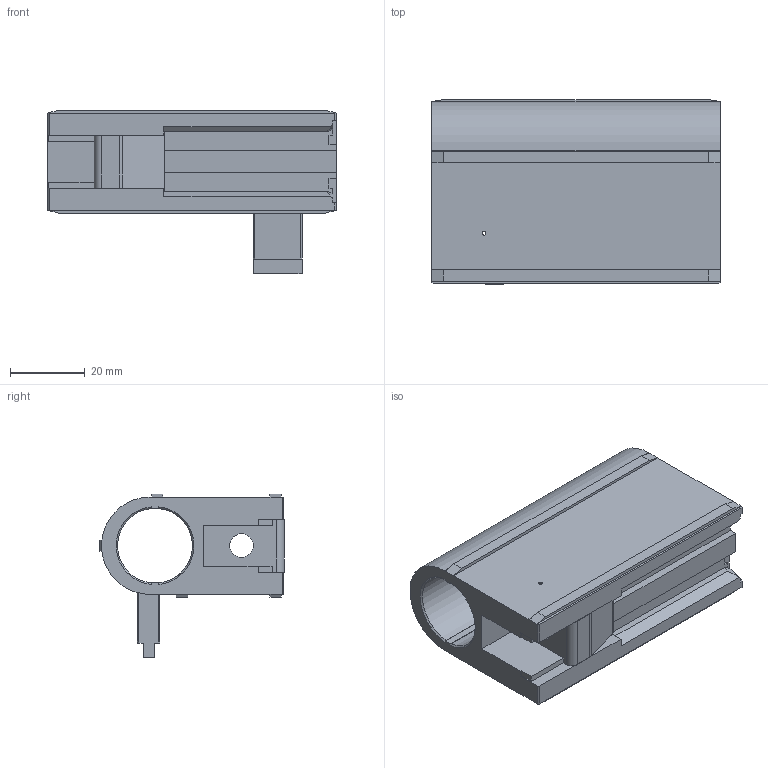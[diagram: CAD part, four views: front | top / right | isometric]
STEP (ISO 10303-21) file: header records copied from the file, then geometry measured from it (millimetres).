
FILE_DESCRIPTION (( 'STEP AP203' ), '1' );
FILE_NAME ('MOD9_bolt_housing.STEP', '2020-06-10T04:56:02', ( '' ), ( '' ), 'SwSTEP 2.0', 'SolidWorks 2016', '' );
FILE_SCHEMA (( 'CONFIG_CONTROL_DESIGN' ));
Length unit declared in the file: millimetre
Products named in the file (1): MOD9_bolt_housing
Bounding box: 77.19 x 49.15 x 43.8 mm (x, y, z)
Volume: 47408.2 mm3; surface area: 22111.7 mm2
Topology: 1 solids, 1 shells, 140 faces, 391 edges, 255 vertices
Faces by surface type: plane 126, cylinder 12, cone 2
Full cylindrical faces by diameter (mm): 0.968 x2, 2.14 x1, 6.34 x1
Entity records: 4557 total; most frequent: CARTESIAN_POINT 878, ORIENTED_EDGE 774, DIRECTION 692, EDGE_CURVE 387, LINE 350, VECTOR 350, VERTEX_POINT 255, AXIS2_PLACEMENT_3D 171
